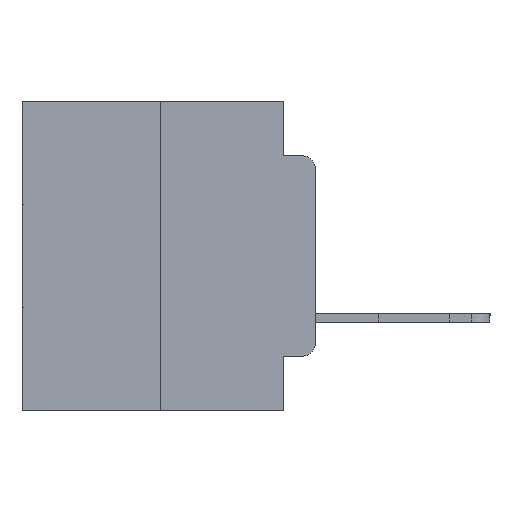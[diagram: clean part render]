
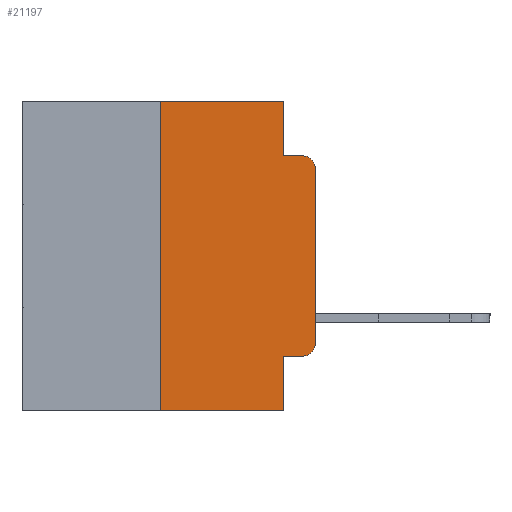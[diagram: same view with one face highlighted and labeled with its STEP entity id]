
A CAD part, left-side view. The second image highlights one B-rep face of the part: STEP entity #21197.
In plain terms, the highlighted planar face has unit normal (-1, 0, 0).
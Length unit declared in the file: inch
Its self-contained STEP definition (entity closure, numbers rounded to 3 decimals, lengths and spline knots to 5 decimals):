
#60 = EDGE_CURVE ( 'NONE', #4696, #5587, #3325, .T. ) ;
#71 = LINE ( 'NONE', #7938, #5541 ) ;
#965 = CARTESIAN_POINT ( 'NONE',  ( 0., 0.051, -0.5 ) ) ;
#1432 = EDGE_CURVE ( 'NONE', #4696, #25556, #12878, .T. ) ;
#1849 = CARTESIAN_POINT ( 'NONE',  ( 0., 0.02, -0.3915 ) ) ;
#2849 = PLANE ( 'NONE',  #21784 ) ;
#3325 = LINE ( 'NONE', #23129, #23574 ) ;
#3596 = ORIENTED_EDGE ( 'NONE', *, *, #60, .T. ) ;
#3896 = DIRECTION ( 'NONE',  ( 0., 0., -1. ) ) ;
#4020 = VECTOR ( 'NONE', #12000, 39.37008 ) ;
#4168 = EDGE_CURVE ( 'NONE', #17658, #26206, #26128, .T. ) ;
#4473 = FACE_OUTER_BOUND ( 'NONE', #23992, .T. ) ;
#4620 = CARTESIAN_POINT ( 'NONE',  ( 0., 0.051, -0.4115 ) ) ;
#4696 = VERTEX_POINT ( 'NONE', #4620 ) ;
#4833 = DIRECTION ( 'NONE',  ( -1., 0., 0. ) ) ;
#4936 = CARTESIAN_POINT ( 'NONE',  ( 0., 0.473, 0. ) ) ;
#5541 = VECTOR ( 'NONE', #23855, 39.37008 ) ;
#5577 = EDGE_CURVE ( 'NONE', #14176, #7163, #18249, .T. ) ;
#5587 = VERTEX_POINT ( 'NONE', #15350 ) ;
#5968 = VECTOR ( 'NONE', #18934, 39.37008 ) ;
#6084 = CARTESIAN_POINT ( 'NONE',  ( 0., 0., -0.3915 ) ) ;
#6926 = EDGE_CURVE ( 'NONE', #7163, #10645, #71, .T. ) ;
#6982 = DIRECTION ( 'NONE',  ( 1., 0., 0. ) ) ;
#7163 = VERTEX_POINT ( 'NONE', #16549 ) ;
#7234 = DIRECTION ( 'NONE',  ( 0., -1., 0. ) ) ;
#7353 = CARTESIAN_POINT ( 'NONE',  ( 0., 0., -0.1085 ) ) ;
#7550 = VECTOR ( 'NONE', #17346, 39.37008 ) ;
#7573 = ORIENTED_EDGE ( 'NONE', *, *, #24986, .T. ) ;
#7938 = CARTESIAN_POINT ( 'NONE',  ( 0., 0.051, -0.0885 ) ) ;
#8915 = CARTESIAN_POINT ( 'NONE',  ( 0., 0., 0. ) ) ;
#9175 = AXIS2_PLACEMENT_3D ( 'NONE', #16942, #4833, #18991 ) ;
#9345 = ORIENTED_EDGE ( 'NONE', *, *, #9710, .T. ) ;
#9479 = VECTOR ( 'NONE', #18756, 39.37008 ) ;
#9710 = EDGE_CURVE ( 'NONE', #16155, #10645, #18698, .T. ) ;
#9768 = ORIENTED_EDGE ( 'NONE', *, *, #15765, .F. ) ;
#9836 = CARTESIAN_POINT ( 'NONE',  ( 0., 0.25, 0. ) ) ;
#9928 = LINE ( 'NONE', #22140, #14664 ) ;
#10645 = VERTEX_POINT ( 'NONE', #11623 ) ;
#10969 = CARTESIAN_POINT ( 'NONE',  ( 0., 0.25, -0.5 ) ) ;
#11090 = EDGE_CURVE ( 'NONE', #11488, #16155, #16712, .T. ) ;
#11488 = VERTEX_POINT ( 'NONE', #6084 ) ;
#11623 = CARTESIAN_POINT ( 'NONE',  ( 0., 0.02, -0.0885 ) ) ;
#11955 = ORIENTED_EDGE ( 'NONE', *, *, #4168, .F. ) ;
#12000 = DIRECTION ( 'NONE',  ( 0., 0., 1. ) ) ;
#12302 = ORIENTED_EDGE ( 'NONE', *, *, #12766, .T. ) ;
#12766 = EDGE_CURVE ( 'NONE', #17658, #25556, #20112, .T. ) ;
#12863 = AXIS2_PLACEMENT_3D ( 'NONE', #1849, #16062, #3896 ) ;
#12878 = LINE ( 'NONE', #24902, #17534 ) ;
#14176 = VERTEX_POINT ( 'NONE', #19952 ) ;
#14664 = VECTOR ( 'NONE', #26167, 39.37008 ) ;
#15350 = CARTESIAN_POINT ( 'NONE',  ( 0., 0.02, -0.4115 ) ) ;
#15765 = EDGE_CURVE ( 'NONE', #26206, #14176, #9928, .T. ) ;
#16062 = DIRECTION ( 'NONE',  ( -1., 0., 0. ) ) ;
#16155 = VERTEX_POINT ( 'NONE', #7353 ) ;
#16458 = ORIENTED_EDGE ( 'NONE', *, *, #11090, .T. ) ;
#16549 = CARTESIAN_POINT ( 'NONE',  ( 0., 0.051, -0.0885 ) ) ;
#16712 = LINE ( 'NONE', #8915, #5968 ) ;
#16713 = CARTESIAN_POINT ( 'NONE',  ( 0., 0.473, -0.5 ) ) ;
#16942 = CARTESIAN_POINT ( 'NONE',  ( 0., 0.02, -0.1085 ) ) ;
#17044 = ORIENTED_EDGE ( 'NONE', *, *, #6926, .F. ) ;
#17346 = DIRECTION ( 'NONE',  ( 0., 0., -1. ) ) ;
#17534 = VECTOR ( 'NONE', #18027, 39.37008 ) ;
#17658 = VERTEX_POINT ( 'NONE', #10969 ) ;
#18027 = DIRECTION ( 'NONE',  ( 0., 0., -1. ) ) ;
#18249 = LINE ( 'NONE', #19298, #7550 ) ;
#18698 = CIRCLE ( 'NONE', #9175, 0.02 ) ;
#18756 = DIRECTION ( 'NONE',  ( 0., -1., 0. ) ) ;
#18934 = DIRECTION ( 'NONE',  ( 0., 0., 1. ) ) ;
#18991 = DIRECTION ( 'NONE',  ( 0., 0., -1. ) ) ;
#19298 = CARTESIAN_POINT ( 'NONE',  ( 0., 0.051, 0. ) ) ;
#19952 = CARTESIAN_POINT ( 'NONE',  ( 0., 0.051, 0. ) ) ;
#20084 = ORIENTED_EDGE ( 'NONE', *, *, #1432, .F. ) ;
#20112 = LINE ( 'NONE', #16713, #9479 ) ;
#21067 = DIRECTION ( 'NONE',  ( 0., 0., -1. ) ) ;
#21197 = ADVANCED_FACE ( 'NONE', ( #4473 ), #2849, .F. ) ;
#21784 = AXIS2_PLACEMENT_3D ( 'NONE', #4936, #6982, #21067 ) ;
#22140 = CARTESIAN_POINT ( 'NONE',  ( 0., 0.473, 0. ) ) ;
#23129 = CARTESIAN_POINT ( 'NONE',  ( 0., 0.051, -0.4115 ) ) ;
#23270 = CIRCLE ( 'NONE', #12863, 0.02 ) ;
#23399 = CARTESIAN_POINT ( 'NONE',  ( 0., 0.25, 0. ) ) ;
#23574 = VECTOR ( 'NONE', #7234, 39.37008 ) ;
#23855 = DIRECTION ( 'NONE',  ( 0., -1., 0. ) ) ;
#23992 = EDGE_LOOP ( 'NONE', ( #16458, #9345, #17044, #25840, #9768, #11955, #12302, #20084, #3596, #7573 ) ) ;
#24902 = CARTESIAN_POINT ( 'NONE',  ( 0., 0.051, 0. ) ) ;
#24986 = EDGE_CURVE ( 'NONE', #5587, #11488, #23270, .T. ) ;
#25556 = VERTEX_POINT ( 'NONE', #965 ) ;
#25840 = ORIENTED_EDGE ( 'NONE', *, *, #5577, .F. ) ;
#26128 = LINE ( 'NONE', #9836, #4020 ) ;
#26167 = DIRECTION ( 'NONE',  ( 0., -1., 0. ) ) ;
#26206 = VERTEX_POINT ( 'NONE', #23399 ) ;
